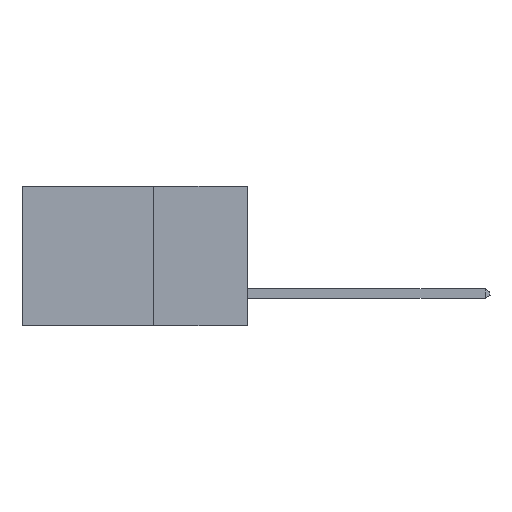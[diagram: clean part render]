
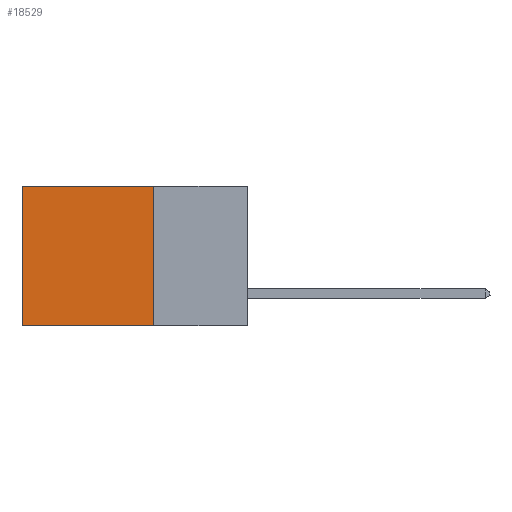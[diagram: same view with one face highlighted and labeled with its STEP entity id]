
A CAD part, left-side view. The second image highlights one B-rep face of the part: STEP entity #18529.
In plain terms, the highlighted planar face has unit normal (-1, 0, 0).
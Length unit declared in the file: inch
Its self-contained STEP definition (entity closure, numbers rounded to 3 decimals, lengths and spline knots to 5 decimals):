
#393 = VECTOR ( 'NONE', #630, 39.37008 ) ;
#569 = VERTEX_POINT ( 'NONE', #9267 ) ;
#580 = VECTOR ( 'NONE', #21603, 39.37008 ) ;
#630 = DIRECTION ( 'NONE',  ( 0., 0., -1. ) ) ;
#867 = ORIENTED_EDGE ( 'NONE', *, *, #22534, .F. ) ;
#1759 = ORIENTED_EDGE ( 'NONE', *, *, #3684, .T. ) ;
#2220 = CARTESIAN_POINT ( 'NONE',  ( 0.298, 0.6, 0. ) ) ;
#2738 = CARTESIAN_POINT ( 'NONE',  ( 0.298, 0.25, 0. ) ) ;
#3112 = DIRECTION ( 'NONE',  ( 0., 0., -1. ) ) ;
#3684 = EDGE_CURVE ( 'NONE', #5154, #20900, #16978, .T. ) ;
#4267 = VECTOR ( 'NONE', #10513, 39.37008 ) ;
#5154 = VERTEX_POINT ( 'NONE', #9415 ) ;
#7002 = DIRECTION ( 'NONE',  ( 1., 0., 0. ) ) ;
#8938 = EDGE_CURVE ( 'NONE', #5154, #16117, #10857, .T. ) ;
#9267 = CARTESIAN_POINT ( 'NONE',  ( 0.298, 0.6, -0.37 ) ) ;
#9415 = CARTESIAN_POINT ( 'NONE',  ( 0.298, 0.25, 0. ) ) ;
#10247 = CARTESIAN_POINT ( 'NONE',  ( 0.298, 0.25, 0. ) ) ;
#10513 = DIRECTION ( 'NONE',  ( 0., 0., -1. ) ) ;
#10736 = CARTESIAN_POINT ( 'NONE',  ( 0.298, 0.25, -0.37 ) ) ;
#10857 = LINE ( 'NONE', #2738, #4267 ) ;
#12789 = EDGE_LOOP ( 'NONE', ( #19135, #867, #22732, #1759 ) ) ;
#12944 = LINE ( 'NONE', #10736, #580 ) ;
#14131 = CARTESIAN_POINT ( 'NONE',  ( 0.298, 0.25, 0. ) ) ;
#15646 = AXIS2_PLACEMENT_3D ( 'NONE', #14131, #7002, #3112 ) ;
#15687 = EDGE_CURVE ( 'NONE', #20900, #569, #20551, .T. ) ;
#16117 = VERTEX_POINT ( 'NONE', #17710 ) ;
#16978 = LINE ( 'NONE', #10247, #17540 ) ;
#17037 = CARTESIAN_POINT ( 'NONE',  ( 0.298, 0.6, 0. ) ) ;
#17540 = VECTOR ( 'NONE', #21202, 39.37008 ) ;
#17710 = CARTESIAN_POINT ( 'NONE',  ( 0.298, 0.25, -0.37 ) ) ;
#17949 = PLANE ( 'NONE',  #15646 ) ;
#18529 = ADVANCED_FACE ( 'NONE', ( #18558 ), #17949, .F. ) ;
#18558 = FACE_OUTER_BOUND ( 'NONE', #12789, .T. ) ;
#19135 = ORIENTED_EDGE ( 'NONE', *, *, #15687, .T. ) ;
#20551 = LINE ( 'NONE', #17037, #393 ) ;
#20900 = VERTEX_POINT ( 'NONE', #2220 ) ;
#21202 = DIRECTION ( 'NONE',  ( 0., 1., 0. ) ) ;
#21603 = DIRECTION ( 'NONE',  ( 0., 1., 0. ) ) ;
#22534 = EDGE_CURVE ( 'NONE', #16117, #569, #12944, .T. ) ;
#22732 = ORIENTED_EDGE ( 'NONE', *, *, #8938, .F. ) ;
